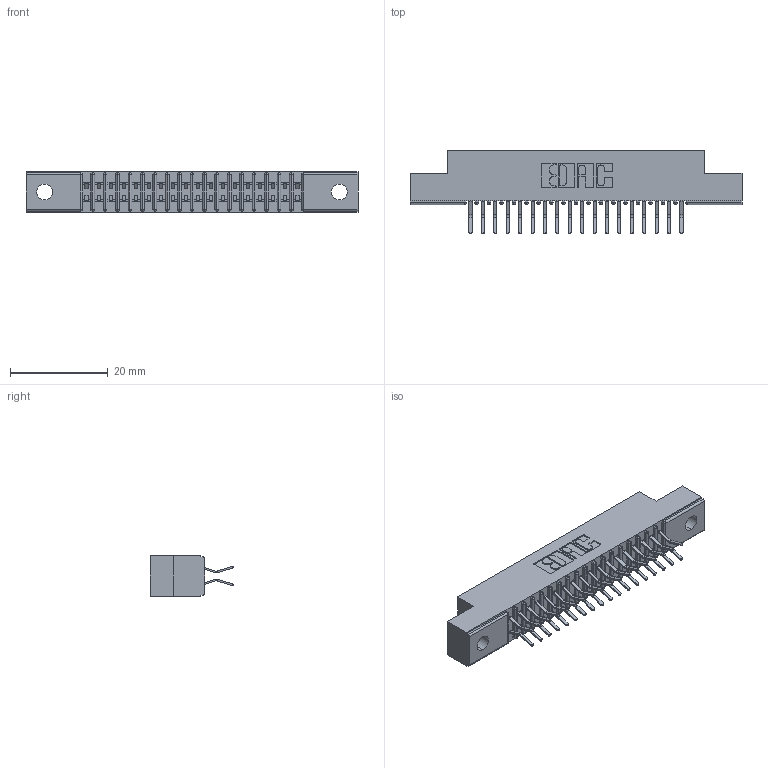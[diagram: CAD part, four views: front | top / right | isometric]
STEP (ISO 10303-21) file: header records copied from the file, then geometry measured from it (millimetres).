
FILE_DESCRIPTION (( 'STEP AP203' ), '1' );
FILE_NAME ('391-036-556-202.STEP', '2018-08-08T23:39:50', ( '' ), ( '' ), 'SwSTEP 2.0', 'SolidWorks 2016', '' );
FILE_SCHEMA (( 'CONFIG_CONTROL_DESIGN' ));
Length unit declared in the file: inch
Products named in the file (3): 341 Part_.128 (3.25) Dia Mounting Holes; 341-292-001_341-292-156; 391-036-556-202
Assembly tree (37 placements, depth 2):
  391-036-556-202
    341 Part_.128 (3.25) Dia Mounting Holes
    341-292-001_341-292-156  x36
Bounding box: 67.94 x 17.07 x 8.38 mm (x, y, z)
Volume: 3850.4 mm3; surface area: 7617.3 mm2
Topology: 37 solids, 37 shells, 2636 faces, 7642 edges, 4958 vertices
Faces by surface type: plane 1508, cylinder 1056, sphere 38, torus 34
Entity records: 25123 total; most frequent: CARTESIAN_POINT 4178, ORIENTED_EDGE 4148, DIRECTION 4076, EDGE_CURVE 2074, VECTOR 1644, LINE 1644, VERTEX_POINT 1318, AXIS2_PLACEMENT_3D 1216
